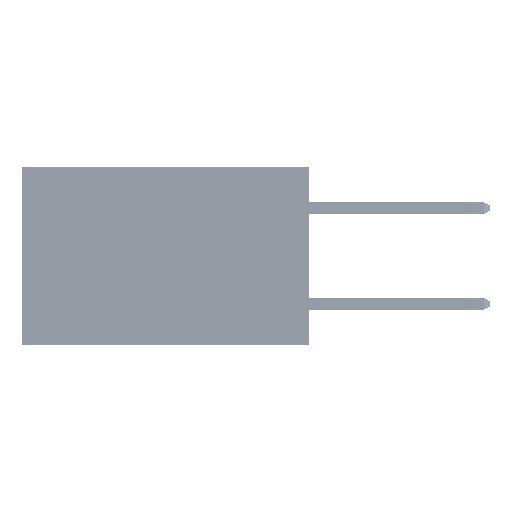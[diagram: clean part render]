
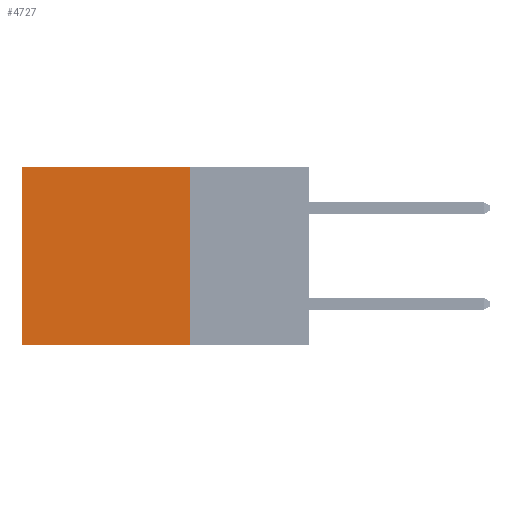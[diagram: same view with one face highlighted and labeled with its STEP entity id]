
A CAD part, left-side view. The second image highlights one B-rep face of the part: STEP entity #4727.
In plain terms, the highlighted planar face has unit normal (-1, 0, 0).
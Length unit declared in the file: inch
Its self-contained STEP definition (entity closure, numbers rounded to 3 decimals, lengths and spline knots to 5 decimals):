
#1283 = DIRECTION ( 'NONE',  ( 0., 0., -1. ) ) ;
#1481 = DIRECTION ( 'NONE',  ( 0., 0., -1. ) ) ;
#2441 = DIRECTION ( 'NONE',  ( 1., 0., 0. ) ) ;
#4588 = EDGE_CURVE ( 'NONE', #21964, #32290, #49491, .T. ) ;
#4727 = ADVANCED_FACE ( 'NONE', ( #22280 ), #15420, .F. ) ;
#8059 = CARTESIAN_POINT ( 'NONE',  ( 0.2875, 0.6, -0.37 ) ) ;
#9448 = VECTOR ( 'NONE', #1283, 39.37008 ) ;
#9847 = CARTESIAN_POINT ( 'NONE',  ( 0.2875, 0.6, 0. ) ) ;
#10016 = DIRECTION ( 'NONE',  ( 0., 1., 0. ) ) ;
#10350 = CARTESIAN_POINT ( 'NONE',  ( 0.2875, 0.25, 0. ) ) ;
#10835 = LINE ( 'NONE', #14738, #12552 ) ;
#10888 = ORIENTED_EDGE ( 'NONE', *, *, #4588, .T. ) ;
#11616 = VECTOR ( 'NONE', #10016, 39.37008 ) ;
#12278 = ORIENTED_EDGE ( 'NONE', *, *, #15782, .F. ) ;
#12552 = VECTOR ( 'NONE', #35112, 39.37008 ) ;
#14738 = CARTESIAN_POINT ( 'NONE',  ( 0.2875, 0.25, -0.37 ) ) ;
#15420 = PLANE ( 'NONE',  #24118 ) ;
#15782 = EDGE_CURVE ( 'NONE', #18591, #40365, #10835, .T. ) ;
#17231 = ORIENTED_EDGE ( 'NONE', *, *, #43032, .T. ) ;
#17943 = CARTESIAN_POINT ( 'NONE',  ( 0.2875, 0.25, -0.37 ) ) ;
#18591 = VERTEX_POINT ( 'NONE', #17943 ) ;
#18689 = LINE ( 'NONE', #26776, #9448 ) ;
#20207 = ORIENTED_EDGE ( 'NONE', *, *, #44855, .F. ) ;
#21964 = VERTEX_POINT ( 'NONE', #39424 ) ;
#22280 = FACE_OUTER_BOUND ( 'NONE', #26462, .T. ) ;
#24118 = AXIS2_PLACEMENT_3D ( 'NONE', #35533, #2441, #39984 ) ;
#26462 = EDGE_LOOP ( 'NONE', ( #17231, #12278, #20207, #10888 ) ) ;
#26776 = CARTESIAN_POINT ( 'NONE',  ( 0.2875, 0.6, 0. ) ) ;
#30375 = VECTOR ( 'NONE', #1481, 39.37008 ) ;
#32290 = VERTEX_POINT ( 'NONE', #9847 ) ;
#35112 = DIRECTION ( 'NONE',  ( 0., 1., 0. ) ) ;
#35533 = CARTESIAN_POINT ( 'NONE',  ( 0.2875, 0.25, 0. ) ) ;
#39424 = CARTESIAN_POINT ( 'NONE',  ( 0.2875, 0.25, 0. ) ) ;
#39984 = DIRECTION ( 'NONE',  ( 0., 0., -1. ) ) ;
#40365 = VERTEX_POINT ( 'NONE', #8059 ) ;
#40882 = CARTESIAN_POINT ( 'NONE',  ( 0.2875, 0.25, 0. ) ) ;
#43032 = EDGE_CURVE ( 'NONE', #32290, #40365, #18689, .T. ) ;
#44855 = EDGE_CURVE ( 'NONE', #21964, #18591, #46153, .T. ) ;
#46153 = LINE ( 'NONE', #10350, #30375 ) ;
#49491 = LINE ( 'NONE', #40882, #11616 ) ;
